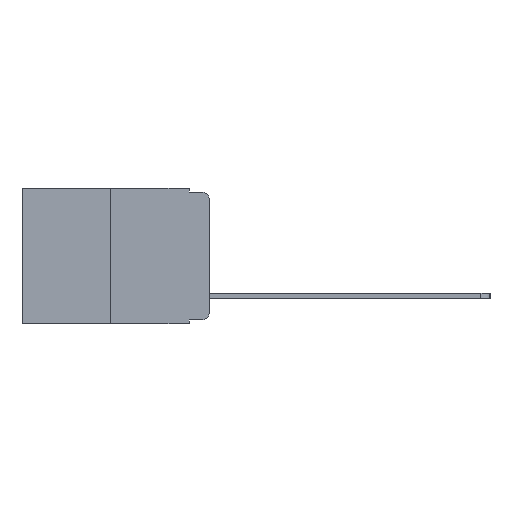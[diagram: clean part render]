
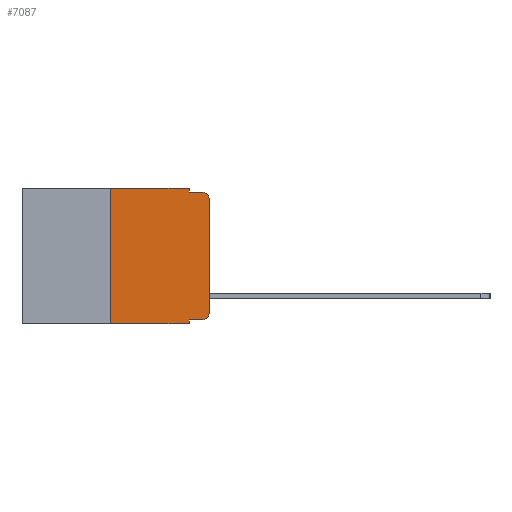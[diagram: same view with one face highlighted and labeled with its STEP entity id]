
A CAD part, left-side view. The second image highlights one B-rep face of the part: STEP entity #7087.
In plain terms, the highlighted planar face has unit normal (-1, 0, 0).
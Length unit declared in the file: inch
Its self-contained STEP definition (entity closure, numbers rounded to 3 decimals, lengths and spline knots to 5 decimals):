
#51 = CARTESIAN_POINT ( 'NONE',  ( 0., 0.051, -0.333 ) ) ;
#160 = LINE ( 'NONE', #6367, #11082 ) ;
#529 = PLANE ( 'NONE',  #12374 ) ;
#650 = CARTESIAN_POINT ( 'NONE',  ( 0., 0., -0.03 ) ) ;
#898 = DIRECTION ( 'NONE',  ( 0., 0., 1. ) ) ;
#937 = CARTESIAN_POINT ( 'NONE',  ( 0., 0.051, -0.01 ) ) ;
#1018 = ORIENTED_EDGE ( 'NONE', *, *, #8789, .F. ) ;
#1204 = DIRECTION ( 'NONE',  ( 0., -1., 0. ) ) ;
#1371 = VERTEX_POINT ( 'NONE', #3262 ) ;
#1574 = EDGE_CURVE ( 'NONE', #1371, #9406, #5590, .T. ) ;
#1626 = DIRECTION ( 'NONE',  ( 1., 0., 0. ) ) ;
#1775 = EDGE_CURVE ( 'NONE', #1371, #13376, #5395, .T. ) ;
#1863 = AXIS2_PLACEMENT_3D ( 'NONE', #2886, #10249, #3997 ) ;
#1957 = LINE ( 'NONE', #51, #12640 ) ;
#2154 = DIRECTION ( 'NONE',  ( 0., 0., -1. ) ) ;
#2512 = ORIENTED_EDGE ( 'NONE', *, *, #8943, .T. ) ;
#2645 = DIRECTION ( 'NONE',  ( 0., 0., 1. ) ) ;
#2853 = CARTESIAN_POINT ( 'NONE',  ( 0., 0.02, -0.01 ) ) ;
#2886 = CARTESIAN_POINT ( 'NONE',  ( 0., 0.02, -0.03 ) ) ;
#3225 = CARTESIAN_POINT ( 'NONE',  ( 0., 0.051, 0. ) ) ;
#3244 = VERTEX_POINT ( 'NONE', #2853 ) ;
#3262 = CARTESIAN_POINT ( 'NONE',  ( 0., 0.25, -0.343 ) ) ;
#3333 = VECTOR ( 'NONE', #8303, 39.37008 ) ;
#3384 = ORIENTED_EDGE ( 'NONE', *, *, #1574, .T. ) ;
#3618 = ORIENTED_EDGE ( 'NONE', *, *, #7846, .T. ) ;
#3646 = VECTOR ( 'NONE', #12456, 39.37008 ) ;
#3683 = FACE_OUTER_BOUND ( 'NONE', #6488, .T. ) ;
#3877 = CARTESIAN_POINT ( 'NONE',  ( 0., 0.051, 0. ) ) ;
#3933 = EDGE_CURVE ( 'NONE', #11485, #8503, #160, .T. ) ;
#3997 = DIRECTION ( 'NONE',  ( 0., 0., -1. ) ) ;
#4168 = LINE ( 'NONE', #5738, #12349 ) ;
#4224 = CARTESIAN_POINT ( 'NONE',  ( 0., 0.02, -0.313 ) ) ;
#4281 = ORIENTED_EDGE ( 'NONE', *, *, #9670, .F. ) ;
#4471 = CARTESIAN_POINT ( 'NONE',  ( 0., 0.25, 0. ) ) ;
#4545 = CIRCLE ( 'NONE', #1863, 0.02 ) ;
#4549 = VERTEX_POINT ( 'NONE', #8274 ) ;
#5096 = ORIENTED_EDGE ( 'NONE', *, *, #6170, .T. ) ;
#5111 = CARTESIAN_POINT ( 'NONE',  ( 0., 0., -0.313 ) ) ;
#5370 = DIRECTION ( 'NONE',  ( 0., 0., -1. ) ) ;
#5395 = LINE ( 'NONE', #11967, #12785 ) ;
#5590 = LINE ( 'NONE', #5937, #8373 ) ;
#5738 = CARTESIAN_POINT ( 'NONE',  ( 0., 0.051, -0.01 ) ) ;
#5937 = CARTESIAN_POINT ( 'NONE',  ( 0., 0.473, -0.343 ) ) ;
#6170 = EDGE_CURVE ( 'NONE', #8970, #11485, #12411, .T. ) ;
#6202 = CARTESIAN_POINT ( 'NONE',  ( 0., 0.051, 0. ) ) ;
#6367 = CARTESIAN_POINT ( 'NONE',  ( 0., 0., 0. ) ) ;
#6461 = ORIENTED_EDGE ( 'NONE', *, *, #7191, .F. ) ;
#6488 = EDGE_LOOP ( 'NONE', ( #11934, #3618, #8466, #4281, #1018, #8624, #3384, #6461, #2512, #5096 ) ) ;
#6998 = DIRECTION ( 'NONE',  ( 0., -1., 0. ) ) ;
#7087 = ADVANCED_FACE ( 'NONE', ( #3683 ), #529, .F. ) ;
#7108 = LINE ( 'NONE', #3225, #9422 ) ;
#7191 = EDGE_CURVE ( 'NONE', #4549, #9406, #8098, .T. ) ;
#7774 = CARTESIAN_POINT ( 'NONE',  ( 0., 0.02, -0.333 ) ) ;
#7846 = EDGE_CURVE ( 'NONE', #8503, #3244, #4545, .T. ) ;
#8098 = LINE ( 'NONE', #6202, #3333 ) ;
#8274 = CARTESIAN_POINT ( 'NONE',  ( 0., 0.051, -0.333 ) ) ;
#8303 = DIRECTION ( 'NONE',  ( 0., 0., -1. ) ) ;
#8373 = VECTOR ( 'NONE', #6998, 39.37008 ) ;
#8466 = ORIENTED_EDGE ( 'NONE', *, *, #9036, .F. ) ;
#8503 = VERTEX_POINT ( 'NONE', #650 ) ;
#8624 = ORIENTED_EDGE ( 'NONE', *, *, #1775, .F. ) ;
#8789 = EDGE_CURVE ( 'NONE', #13376, #10907, #11891, .T. ) ;
#8943 = EDGE_CURVE ( 'NONE', #4549, #8970, #1957, .T. ) ;
#8970 = VERTEX_POINT ( 'NONE', #7774 ) ;
#9036 = EDGE_CURVE ( 'NONE', #12113, #3244, #4168, .T. ) ;
#9129 = DIRECTION ( 'NONE',  ( 0., 0., -1. ) ) ;
#9406 = VERTEX_POINT ( 'NONE', #12204 ) ;
#9422 = VECTOR ( 'NONE', #2154, 39.37008 ) ;
#9670 = EDGE_CURVE ( 'NONE', #10907, #12113, #7108, .T. ) ;
#10249 = DIRECTION ( 'NONE',  ( -1., 0., 0. ) ) ;
#10907 = VERTEX_POINT ( 'NONE', #3877 ) ;
#10962 = AXIS2_PLACEMENT_3D ( 'NONE', #4224, #11436, #5370 ) ;
#11023 = CARTESIAN_POINT ( 'NONE',  ( 0., 0.473, 0. ) ) ;
#11082 = VECTOR ( 'NONE', #898, 39.37008 ) ;
#11436 = DIRECTION ( 'NONE',  ( -1., 0., 0. ) ) ;
#11472 = CARTESIAN_POINT ( 'NONE',  ( 0., 0.473, 0. ) ) ;
#11485 = VERTEX_POINT ( 'NONE', #5111 ) ;
#11758 = DIRECTION ( 'NONE',  ( 0., -1., 0. ) ) ;
#11891 = LINE ( 'NONE', #11472, #3646 ) ;
#11934 = ORIENTED_EDGE ( 'NONE', *, *, #3933, .T. ) ;
#11967 = CARTESIAN_POINT ( 'NONE',  ( 0., 0.25, 0. ) ) ;
#12113 = VERTEX_POINT ( 'NONE', #937 ) ;
#12204 = CARTESIAN_POINT ( 'NONE',  ( 0., 0.051, -0.343 ) ) ;
#12349 = VECTOR ( 'NONE', #11758, 39.37008 ) ;
#12374 = AXIS2_PLACEMENT_3D ( 'NONE', #11023, #1626, #9129 ) ;
#12411 = CIRCLE ( 'NONE', #10962, 0.02 ) ;
#12456 = DIRECTION ( 'NONE',  ( 0., -1., 0. ) ) ;
#12640 = VECTOR ( 'NONE', #1204, 39.37008 ) ;
#12785 = VECTOR ( 'NONE', #2645, 39.37008 ) ;
#13376 = VERTEX_POINT ( 'NONE', #4471 ) ;
